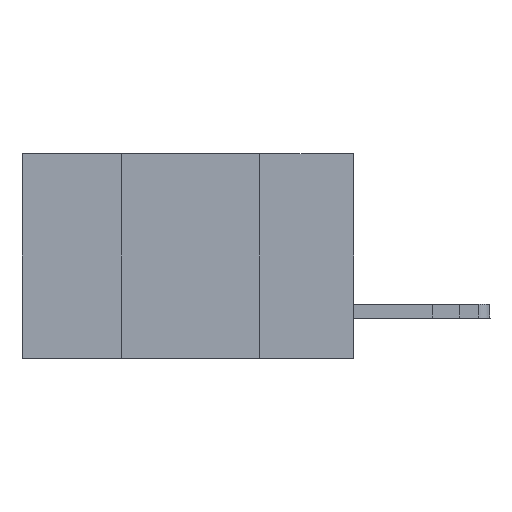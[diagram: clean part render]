
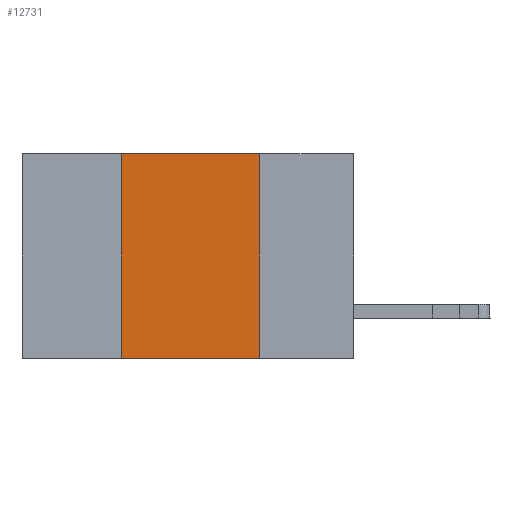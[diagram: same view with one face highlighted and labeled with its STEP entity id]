
A CAD part, left-side view. The second image highlights one B-rep face of the part: STEP entity #12731.
In plain terms, the highlighted planar face has unit normal (-1, 0, 0).
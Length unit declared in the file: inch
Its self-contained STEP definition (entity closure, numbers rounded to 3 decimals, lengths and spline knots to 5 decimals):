
#100 = VECTOR ( 'NONE', #4195, 39.37008 ) ;
#950 = LINE ( 'NONE', #8980, #10841 ) ;
#1048 = DIRECTION ( 'NONE',  ( 0., 0., -1. ) ) ;
#1657 = DIRECTION ( 'NONE',  ( 1., 0., 0. ) ) ;
#4081 = CARTESIAN_POINT ( 'NONE',  ( 0., 0.6, 0. ) ) ;
#4195 = DIRECTION ( 'NONE',  ( 0., -1., 0. ) ) ;
#4377 = EDGE_CURVE ( 'NONE', #9315, #8185, #13219, .T. ) ;
#5155 = ORIENTED_EDGE ( 'NONE', *, *, #10279, .F. ) ;
#5582 = CARTESIAN_POINT ( 'NONE',  ( 0., 0.6, -0.37 ) ) ;
#5635 = ORIENTED_EDGE ( 'NONE', *, *, #4377, .T. ) ;
#6078 = PLANE ( 'NONE',  #7030 ) ;
#6424 = LINE ( 'NONE', #9642, #17910 ) ;
#7030 = AXIS2_PLACEMENT_3D ( 'NONE', #7583, #1657, #9009 ) ;
#7583 = CARTESIAN_POINT ( 'NONE',  ( 0., 0.6, 0. ) ) ;
#8185 = VERTEX_POINT ( 'NONE', #18088 ) ;
#8491 = LINE ( 'NONE', #4081, #9912 ) ;
#8980 = CARTESIAN_POINT ( 'NONE',  ( 0., 0.17, 0. ) ) ;
#9009 = DIRECTION ( 'NONE',  ( 0., 0., -1. ) ) ;
#9315 = VERTEX_POINT ( 'NONE', #12858 ) ;
#9642 = CARTESIAN_POINT ( 'NONE',  ( 0., 0.42, 0. ) ) ;
#9912 = VECTOR ( 'NONE', #13312, 39.37008 ) ;
#10279 = EDGE_CURVE ( 'NONE', #18412, #8185, #950, .T. ) ;
#10841 = VECTOR ( 'NONE', #1048, 39.37008 ) ;
#10885 = EDGE_CURVE ( 'NONE', #9315, #17261, #6424, .T. ) ;
#12731 = ADVANCED_FACE ( 'NONE', ( #15011 ), #6078, .F. ) ;
#12858 = CARTESIAN_POINT ( 'NONE',  ( 0., 0.42, -0.37 ) ) ;
#13021 = EDGE_CURVE ( 'NONE', #17261, #18412, #8491, .T. ) ;
#13219 = LINE ( 'NONE', #5582, #100 ) ;
#13312 = DIRECTION ( 'NONE',  ( 0., -1., 0. ) ) ;
#14256 = DIRECTION ( 'NONE',  ( 0., 0., 1. ) ) ;
#15011 = FACE_OUTER_BOUND ( 'NONE', #16007, .T. ) ;
#15616 = CARTESIAN_POINT ( 'NONE',  ( 0., 0.17, 0. ) ) ;
#16007 = EDGE_LOOP ( 'NONE', ( #5155, #18016, #16399, #5635 ) ) ;
#16399 = ORIENTED_EDGE ( 'NONE', *, *, #10885, .F. ) ;
#16520 = CARTESIAN_POINT ( 'NONE',  ( 0., 0.42, 0. ) ) ;
#17261 = VERTEX_POINT ( 'NONE', #16520 ) ;
#17910 = VECTOR ( 'NONE', #14256, 39.37008 ) ;
#18016 = ORIENTED_EDGE ( 'NONE', *, *, #13021, .F. ) ;
#18088 = CARTESIAN_POINT ( 'NONE',  ( 0., 0.17, -0.37 ) ) ;
#18412 = VERTEX_POINT ( 'NONE', #15616 ) ;
